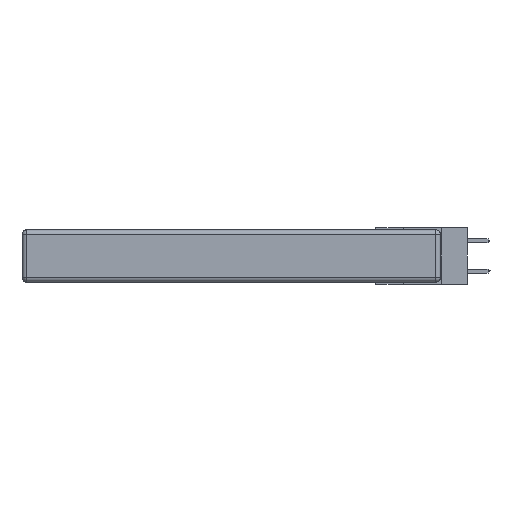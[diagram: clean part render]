
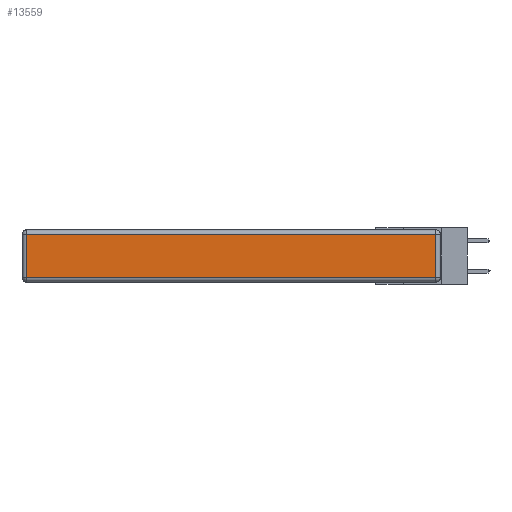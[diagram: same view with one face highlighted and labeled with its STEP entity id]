
A CAD part, left-side view. The second image highlights one B-rep face of the part: STEP entity #13559.
In plain terms, the highlighted planar face has unit normal (-1, 0, 0).
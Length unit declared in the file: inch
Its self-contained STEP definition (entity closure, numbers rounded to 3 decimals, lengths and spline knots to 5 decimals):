
#2385 = EDGE_LOOP ( 'NONE', ( #5184, #33277, #28132, #29539 ) ) ;
#3100 = VERTEX_POINT ( 'NONE', #19915 ) ;
#3457 = LINE ( 'NONE', #9752, #30697 ) ;
#3719 = EDGE_CURVE ( 'NONE', #20666, #3100, #21373, .T. ) ;
#4653 = CARTESIAN_POINT ( 'NONE',  ( 0., 0.03, -0.343 ) ) ;
#5184 = ORIENTED_EDGE ( 'NONE', *, *, #21407, .T. ) ;
#7243 = VECTOR ( 'NONE', #17273, 39.37008 ) ;
#9752 = CARTESIAN_POINT ( 'NONE',  ( 0., 2.72, -0.343 ) ) ;
#10155 = DIRECTION ( 'NONE',  ( 0., 0., 1. ) ) ;
#10689 = CARTESIAN_POINT ( 'NONE',  ( 0., 2.72, -0.313 ) ) ;
#12153 = VECTOR ( 'NONE', #18831, 39.37008 ) ;
#13559 = ADVANCED_FACE ( 'NONE', ( #20189 ), #26119, .T. ) ;
#13745 = VERTEX_POINT ( 'NONE', #10689 ) ;
#15969 = VECTOR ( 'NONE', #30279, 39.37008 ) ;
#16228 = LINE ( 'NONE', #17383, #7243 ) ;
#17273 = DIRECTION ( 'NONE',  ( 0., -1., 0. ) ) ;
#17383 = CARTESIAN_POINT ( 'NONE',  ( 0., 0., -0.313 ) ) ;
#18831 = DIRECTION ( 'NONE',  ( 0., 0., 1. ) ) ;
#19915 = CARTESIAN_POINT ( 'NONE',  ( 0., 2.72, -0.03 ) ) ;
#20189 = FACE_OUTER_BOUND ( 'NONE', #2385, .T. ) ;
#20666 = VERTEX_POINT ( 'NONE', #32762 ) ;
#20840 = EDGE_CURVE ( 'NONE', #27454, #20666, #20857, .T. ) ;
#20857 = LINE ( 'NONE', #4653, #12153 ) ;
#21373 = LINE ( 'NONE', #24970, #15969 ) ;
#21407 = EDGE_CURVE ( 'NONE', #13745, #27454, #16228, .T. ) ;
#22087 = EDGE_CURVE ( 'NONE', #3100, #13745, #3457, .T. ) ;
#23958 = AXIS2_PLACEMENT_3D ( 'NONE', #31196, #28667, #10155 ) ;
#24970 = CARTESIAN_POINT ( 'NONE',  ( 0., 2.75, -0.03 ) ) ;
#26119 = PLANE ( 'NONE',  #23958 ) ;
#27454 = VERTEX_POINT ( 'NONE', #31910 ) ;
#28132 = ORIENTED_EDGE ( 'NONE', *, *, #3719, .T. ) ;
#28667 = DIRECTION ( 'NONE',  ( -1., 0., 0. ) ) ;
#29539 = ORIENTED_EDGE ( 'NONE', *, *, #22087, .T. ) ;
#30279 = DIRECTION ( 'NONE',  ( 0., 1., 0. ) ) ;
#30697 = VECTOR ( 'NONE', #33470, 39.37008 ) ;
#31196 = CARTESIAN_POINT ( 'NONE',  ( 0., 0., -0.343 ) ) ;
#31910 = CARTESIAN_POINT ( 'NONE',  ( 0., 0.03, -0.313 ) ) ;
#32762 = CARTESIAN_POINT ( 'NONE',  ( 0., 0.03, -0.03 ) ) ;
#33277 = ORIENTED_EDGE ( 'NONE', *, *, #20840, .T. ) ;
#33470 = DIRECTION ( 'NONE',  ( 0., 0., -1. ) ) ;
